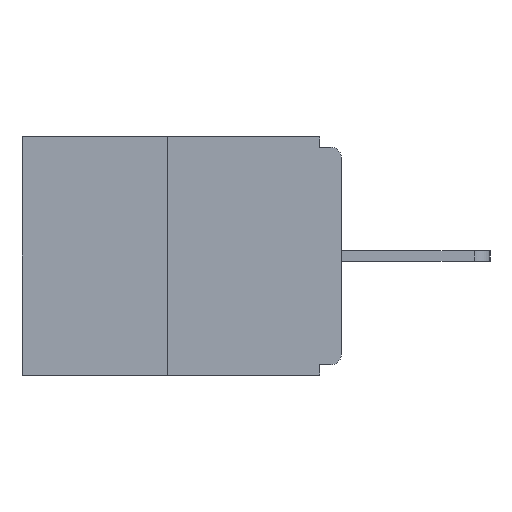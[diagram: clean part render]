
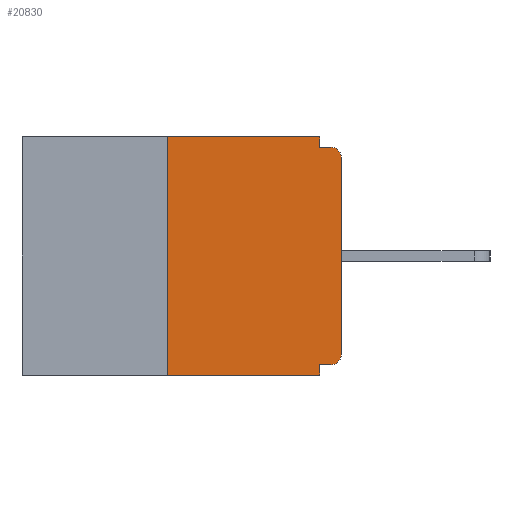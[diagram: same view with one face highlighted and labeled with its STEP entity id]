
A CAD part, left-side view. The second image highlights one B-rep face of the part: STEP entity #20830.
In plain terms, the highlighted planar face has unit normal (-1, 0, 0).
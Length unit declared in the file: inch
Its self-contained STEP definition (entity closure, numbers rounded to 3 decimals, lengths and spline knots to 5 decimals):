
#294 = VERTEX_POINT ( 'NONE', #11990 ) ;
#402 = ORIENTED_EDGE ( 'NONE', *, *, #14048, .F. ) ;
#586 = DIRECTION ( 'NONE',  ( 0., 0., -1. ) ) ;
#670 = AXIS2_PLACEMENT_3D ( 'NONE', #14047, #15535, #12127 ) ;
#1122 = VECTOR ( 'NONE', #6474, 39.37008 ) ;
#1384 = LINE ( 'NONE', #4963, #1122 ) ;
#1634 = VERTEX_POINT ( 'NONE', #11156 ) ;
#1892 = AXIS2_PLACEMENT_3D ( 'NONE', #9237, #13739, #17351 ) ;
#2664 = EDGE_CURVE ( 'NONE', #12260, #294, #19539, .T. ) ;
#3150 = LINE ( 'NONE', #19464, #19973 ) ;
#3327 = DIRECTION ( 'NONE',  ( 0., 0., 1. ) ) ;
#3358 = EDGE_CURVE ( 'NONE', #12280, #1634, #3150, .T. ) ;
#3693 = CARTESIAN_POINT ( 'NONE',  ( 0., 0., -0.313 ) ) ;
#3926 = DIRECTION ( 'NONE',  ( 0., 1., 0. ) ) ;
#4052 = DIRECTION ( 'NONE',  ( 0., 0., -1. ) ) ;
#4360 = CARTESIAN_POINT ( 'NONE',  ( 0., 0.46, -0.343 ) ) ;
#4504 = CARTESIAN_POINT ( 'NONE',  ( 0., 0.46, 0. ) ) ;
#4676 = VECTOR ( 'NONE', #5420, 39.37008 ) ;
#4798 = CARTESIAN_POINT ( 'NONE',  ( 0., 0.031, -0.015 ) ) ;
#4963 = CARTESIAN_POINT ( 'NONE',  ( 0., 0.46, 0. ) ) ;
#5011 = CARTESIAN_POINT ( 'NONE',  ( 0., 0., 0. ) ) ;
#5406 = VECTOR ( 'NONE', #4052, 39.37008 ) ;
#5420 = DIRECTION ( 'NONE',  ( 0., -1., 0. ) ) ;
#5455 = LINE ( 'NONE', #9079, #6084 ) ;
#5691 = EDGE_CURVE ( 'NONE', #18952, #13153, #15157, .T. ) ;
#5782 = PLANE ( 'NONE',  #7957 ) ;
#6084 = VECTOR ( 'NONE', #586, 39.37008 ) ;
#6474 = DIRECTION ( 'NONE',  ( 0., -1., 0. ) ) ;
#6531 = EDGE_CURVE ( 'NONE', #13153, #20529, #7364, .T. ) ;
#6602 = EDGE_CURVE ( 'NONE', #19676, #14854, #5455, .T. ) ;
#6815 = CARTESIAN_POINT ( 'NONE',  ( 0., 0., -0.015 ) ) ;
#6842 = VECTOR ( 'NONE', #15911, 39.37008 ) ;
#7211 = ORIENTED_EDGE ( 'NONE', *, *, #6531, .F. ) ;
#7364 = LINE ( 'NONE', #12088, #5406 ) ;
#7957 = AXIS2_PLACEMENT_3D ( 'NONE', #4504, #17216, #12310 ) ;
#8307 = EDGE_CURVE ( 'NONE', #12280, #20529, #15809, .T. ) ;
#8474 = CARTESIAN_POINT ( 'NONE',  ( 0., 0.031, 0. ) ) ;
#8694 = ORIENTED_EDGE ( 'NONE', *, *, #9941, .T. ) ;
#8735 = CARTESIAN_POINT ( 'NONE',  ( 0., 0., -0.328 ) ) ;
#8823 = ORIENTED_EDGE ( 'NONE', *, *, #8307, .T. ) ;
#9079 = CARTESIAN_POINT ( 'NONE',  ( 0., 0.031, 0. ) ) ;
#9204 = CARTESIAN_POINT ( 'NONE',  ( 0., 0.015, -0.015 ) ) ;
#9237 = CARTESIAN_POINT ( 'NONE',  ( 0., 0.015, -0.03 ) ) ;
#9314 = CARTESIAN_POINT ( 'NONE',  ( 0., 0.031, -0.328 ) ) ;
#9389 = EDGE_CURVE ( 'NONE', #14854, #20936, #18147, .T. ) ;
#9629 = EDGE_LOOP ( 'NONE', ( #402, #20570, #8823, #7211, #17304, #8694, #19007, #9928, #15537, #20339 ) ) ;
#9857 = CIRCLE ( 'NONE', #670, 0.015 ) ;
#9928 = ORIENTED_EDGE ( 'NONE', *, *, #18183, .T. ) ;
#9941 = EDGE_CURVE ( 'NONE', #18952, #12260, #9857, .T. ) ;
#10803 = FACE_OUTER_BOUND ( 'NONE', #9629, .T. ) ;
#11156 = CARTESIAN_POINT ( 'NONE',  ( 0., 0.25, 0. ) ) ;
#11990 = CARTESIAN_POINT ( 'NONE',  ( 0., 0., -0.03 ) ) ;
#12088 = CARTESIAN_POINT ( 'NONE',  ( 0., 0.031, -0.343 ) ) ;
#12127 = DIRECTION ( 'NONE',  ( 0., 0., -1. ) ) ;
#12260 = VERTEX_POINT ( 'NONE', #3693 ) ;
#12280 = VERTEX_POINT ( 'NONE', #13641 ) ;
#12310 = DIRECTION ( 'NONE',  ( 0., 0., -1. ) ) ;
#12475 = CARTESIAN_POINT ( 'NONE',  ( 0., 0.015, -0.328 ) ) ;
#12762 = DIRECTION ( 'NONE',  ( 0., 0., 1. ) ) ;
#13153 = VERTEX_POINT ( 'NONE', #9314 ) ;
#13216 = VECTOR ( 'NONE', #3327, 39.37008 ) ;
#13641 = CARTESIAN_POINT ( 'NONE',  ( 0., 0.25, -0.343 ) ) ;
#13739 = DIRECTION ( 'NONE',  ( -1., 0., 0. ) ) ;
#13750 = CARTESIAN_POINT ( 'NONE',  ( 0., 0.031, -0.343 ) ) ;
#14047 = CARTESIAN_POINT ( 'NONE',  ( 0., 0.015, -0.313 ) ) ;
#14048 = EDGE_CURVE ( 'NONE', #1634, #19676, #1384, .T. ) ;
#14854 = VERTEX_POINT ( 'NONE', #4798 ) ;
#15157 = LINE ( 'NONE', #8735, #17028 ) ;
#15535 = DIRECTION ( 'NONE',  ( -1., 0., 0. ) ) ;
#15537 = ORIENTED_EDGE ( 'NONE', *, *, #9389, .F. ) ;
#15809 = LINE ( 'NONE', #4360, #6842 ) ;
#15911 = DIRECTION ( 'NONE',  ( 0., -1., 0. ) ) ;
#17028 = VECTOR ( 'NONE', #3926, 39.37008 ) ;
#17216 = DIRECTION ( 'NONE',  ( 1., 0., 0. ) ) ;
#17304 = ORIENTED_EDGE ( 'NONE', *, *, #5691, .F. ) ;
#17351 = DIRECTION ( 'NONE',  ( 0., 0., -1. ) ) ;
#18147 = LINE ( 'NONE', #6815, #4676 ) ;
#18183 = EDGE_CURVE ( 'NONE', #294, #20936, #19614, .T. ) ;
#18952 = VERTEX_POINT ( 'NONE', #12475 ) ;
#19007 = ORIENTED_EDGE ( 'NONE', *, *, #2664, .T. ) ;
#19464 = CARTESIAN_POINT ( 'NONE',  ( 0., 0.25, 0. ) ) ;
#19539 = LINE ( 'NONE', #5011, #13216 ) ;
#19614 = CIRCLE ( 'NONE', #1892, 0.015 ) ;
#19676 = VERTEX_POINT ( 'NONE', #8474 ) ;
#19973 = VECTOR ( 'NONE', #12762, 39.37008 ) ;
#20339 = ORIENTED_EDGE ( 'NONE', *, *, #6602, .F. ) ;
#20529 = VERTEX_POINT ( 'NONE', #13750 ) ;
#20570 = ORIENTED_EDGE ( 'NONE', *, *, #3358, .F. ) ;
#20830 = ADVANCED_FACE ( 'NONE', ( #10803 ), #5782, .F. ) ;
#20936 = VERTEX_POINT ( 'NONE', #9204 ) ;
